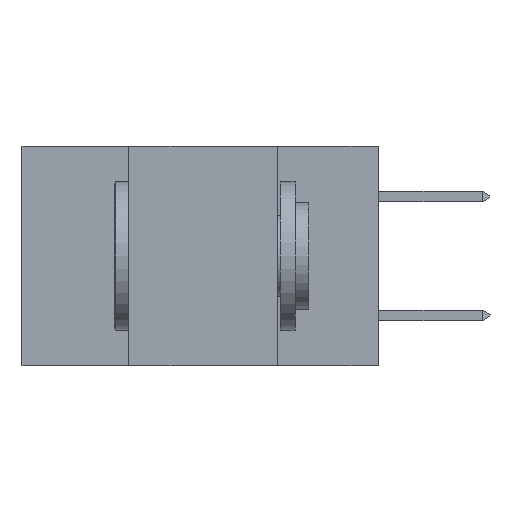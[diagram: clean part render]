
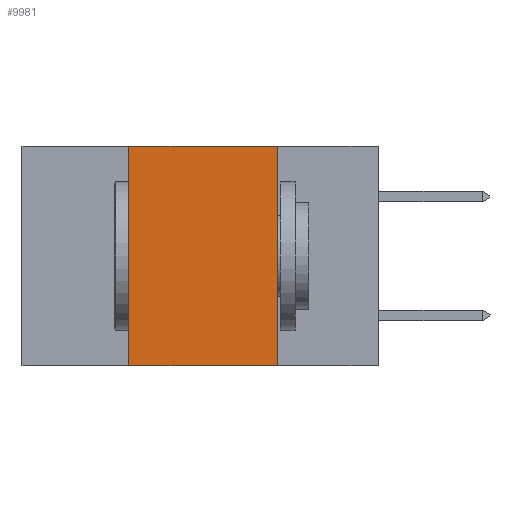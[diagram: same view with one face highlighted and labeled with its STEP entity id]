
A CAD part, left-side view. The second image highlights one B-rep face of the part: STEP entity #9981.
In plain terms, the highlighted planar face has unit normal (-1, 0, 0).
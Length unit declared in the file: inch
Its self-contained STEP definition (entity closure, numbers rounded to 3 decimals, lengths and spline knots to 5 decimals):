
#105 = LINE ( 'NONE', #4473, #779 ) ;
#118 = ORIENTED_EDGE ( 'NONE', *, *, #8254, .T. ) ;
#661 = VECTOR ( 'NONE', #1568, 39.37008 ) ;
#779 = VECTOR ( 'NONE', #8813, 39.37008 ) ;
#932 = EDGE_CURVE ( 'NONE', #3811, #8857, #4496, .T. ) ;
#1036 = VERTEX_POINT ( 'NONE', #5221 ) ;
#1568 = DIRECTION ( 'NONE',  ( 0., -1., 0. ) ) ;
#1808 = DIRECTION ( 'NONE',  ( 1., 0., 0. ) ) ;
#2491 = EDGE_CURVE ( 'NONE', #9874, #1036, #6348, .T. ) ;
#2791 = AXIS2_PLACEMENT_3D ( 'NONE', #5057, #1808, #5921 ) ;
#3120 = CARTESIAN_POINT ( 'NONE',  ( 0., 0.17, 0. ) ) ;
#3310 = CARTESIAN_POINT ( 'NONE',  ( 0., 0.42, -0.37 ) ) ;
#3811 = VERTEX_POINT ( 'NONE', #3120 ) ;
#4095 = VECTOR ( 'NONE', #6031, 39.37008 ) ;
#4325 = ORIENTED_EDGE ( 'NONE', *, *, #932, .F. ) ;
#4473 = CARTESIAN_POINT ( 'NONE',  ( 0., 0.6, -0.37 ) ) ;
#4496 = LINE ( 'NONE', #7224, #9690 ) ;
#4915 = CARTESIAN_POINT ( 'NONE',  ( 0., 0.6, 0. ) ) ;
#5047 = DIRECTION ( 'NONE',  ( 0., 0., -1. ) ) ;
#5057 = CARTESIAN_POINT ( 'NONE',  ( 0., 0.6, 0. ) ) ;
#5221 = CARTESIAN_POINT ( 'NONE',  ( 0., 0.42, 0. ) ) ;
#5504 = PLANE ( 'NONE',  #2791 ) ;
#5574 = LINE ( 'NONE', #4915, #661 ) ;
#5921 = DIRECTION ( 'NONE',  ( 0., 0., -1. ) ) ;
#6031 = DIRECTION ( 'NONE',  ( 0., 0., 1. ) ) ;
#6293 = CARTESIAN_POINT ( 'NONE',  ( 0., 0.17, -0.37 ) ) ;
#6348 = LINE ( 'NONE', #8516, #4095 ) ;
#6768 = ORIENTED_EDGE ( 'NONE', *, *, #2491, .F. ) ;
#7224 = CARTESIAN_POINT ( 'NONE',  ( 0., 0.17, -0.37 ) ) ;
#7947 = EDGE_CURVE ( 'NONE', #1036, #3811, #5574, .T. ) ;
#8254 = EDGE_CURVE ( 'NONE', #9874, #8857, #105, .T. ) ;
#8516 = CARTESIAN_POINT ( 'NONE',  ( 0., 0.42, -0.37 ) ) ;
#8521 = ORIENTED_EDGE ( 'NONE', *, *, #7947, .F. ) ;
#8813 = DIRECTION ( 'NONE',  ( 0., -1., 0. ) ) ;
#8857 = VERTEX_POINT ( 'NONE', #6293 ) ;
#8960 = FACE_OUTER_BOUND ( 'NONE', #10239, .T. ) ;
#9690 = VECTOR ( 'NONE', #5047, 39.37008 ) ;
#9874 = VERTEX_POINT ( 'NONE', #3310 ) ;
#9981 = ADVANCED_FACE ( 'NONE', ( #8960 ), #5504, .F. ) ;
#10239 = EDGE_LOOP ( 'NONE', ( #4325, #8521, #6768, #118 ) ) ;
